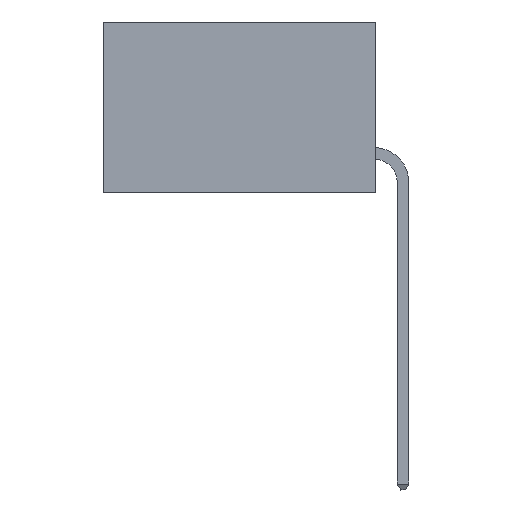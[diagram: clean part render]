
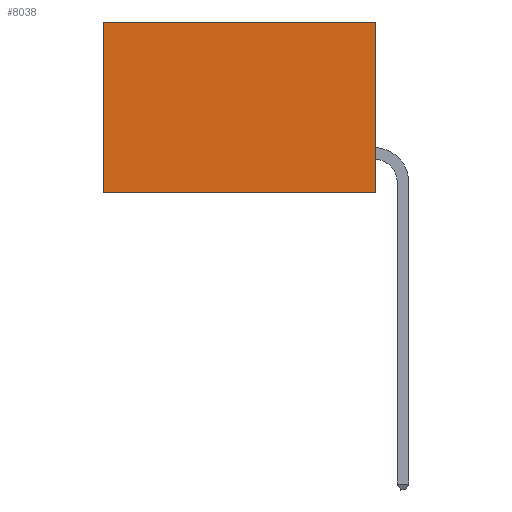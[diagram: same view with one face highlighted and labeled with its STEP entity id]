
A CAD part, left-side view. The second image highlights one B-rep face of the part: STEP entity #8038.
In plain terms, the highlighted planar face has unit normal (-1, 0, 0).
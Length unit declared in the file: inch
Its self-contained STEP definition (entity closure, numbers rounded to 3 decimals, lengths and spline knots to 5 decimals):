
#223 = CARTESIAN_POINT ( 'NONE',  ( 0.277, 0., 0. ) ) ;
#1009 = DIRECTION ( 'NONE',  ( 1., 0., 0. ) ) ;
#1032 = FACE_OUTER_BOUND ( 'NONE', #8644, .T. ) ;
#1104 = VECTOR ( 'NONE', #7617, 39.37008 ) ;
#1209 = ORIENTED_EDGE ( 'NONE', *, *, #3151, .F. ) ;
#1353 = CARTESIAN_POINT ( 'NONE',  ( 0.277, 0., 0. ) ) ;
#1444 = EDGE_CURVE ( 'NONE', #5093, #5086, #8815, .T. ) ;
#1735 = CARTESIAN_POINT ( 'NONE',  ( 0.277, 0.59, 0. ) ) ;
#1773 = VECTOR ( 'NONE', #11559, 39.37008 ) ;
#3043 = EDGE_CURVE ( 'NONE', #6376, #11732, #7586, .T. ) ;
#3066 = CARTESIAN_POINT ( 'NONE',  ( 0.277, 0., -0.37 ) ) ;
#3078 = EDGE_CURVE ( 'NONE', #5086, #11732, #6773, .T. ) ;
#3151 = EDGE_CURVE ( 'NONE', #5093, #6376, #10263, .T. ) ;
#3215 = VECTOR ( 'NONE', #8372, 39.37008 ) ;
#3217 = DIRECTION ( 'NONE',  ( 0., 1., 0. ) ) ;
#4977 = CARTESIAN_POINT ( 'NONE',  ( 0.277, 0., -0.37 ) ) ;
#5086 = VERTEX_POINT ( 'NONE', #1735 ) ;
#5093 = VERTEX_POINT ( 'NONE', #1353 ) ;
#5930 = ORIENTED_EDGE ( 'NONE', *, *, #1444, .T. ) ;
#6345 = ORIENTED_EDGE ( 'NONE', *, *, #3043, .F. ) ;
#6376 = VERTEX_POINT ( 'NONE', #11552 ) ;
#6773 = LINE ( 'NONE', #11742, #1773 ) ;
#6870 = ORIENTED_EDGE ( 'NONE', *, *, #3078, .T. ) ;
#7586 = LINE ( 'NONE', #4977, #9653 ) ;
#7604 = DIRECTION ( 'NONE',  ( 0., 0., -1. ) ) ;
#7617 = DIRECTION ( 'NONE',  ( 0., 1., 0. ) ) ;
#8038 = ADVANCED_FACE ( 'NONE', ( #1032 ), #8421, .F. ) ;
#8372 = DIRECTION ( 'NONE',  ( 0., 0., -1. ) ) ;
#8415 = CARTESIAN_POINT ( 'NONE',  ( 0.277, 0., -0.37 ) ) ;
#8421 = PLANE ( 'NONE',  #9010 ) ;
#8644 = EDGE_LOOP ( 'NONE', ( #6870, #6345, #1209, #5930 ) ) ;
#8815 = LINE ( 'NONE', #223, #1104 ) ;
#9010 = AXIS2_PLACEMENT_3D ( 'NONE', #3066, #1009, #7604 ) ;
#9653 = VECTOR ( 'NONE', #3217, 39.37008 ) ;
#10263 = LINE ( 'NONE', #8415, #3215 ) ;
#10746 = CARTESIAN_POINT ( 'NONE',  ( 0.277, 0.59, -0.37 ) ) ;
#11552 = CARTESIAN_POINT ( 'NONE',  ( 0.277, 0., -0.37 ) ) ;
#11559 = DIRECTION ( 'NONE',  ( 0., 0., -1. ) ) ;
#11732 = VERTEX_POINT ( 'NONE', #10746 ) ;
#11742 = CARTESIAN_POINT ( 'NONE',  ( 0.277, 0.59, -0.37 ) ) ;
